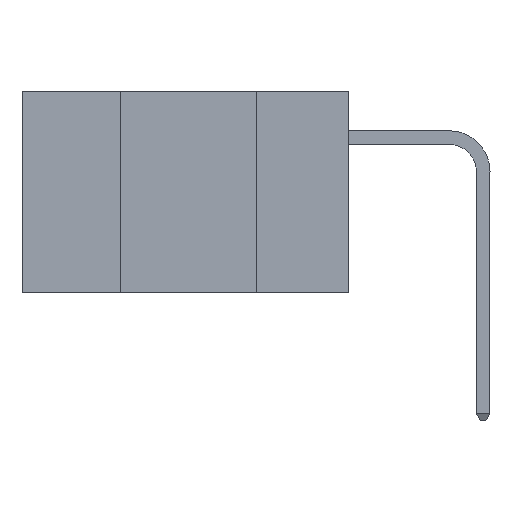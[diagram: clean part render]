
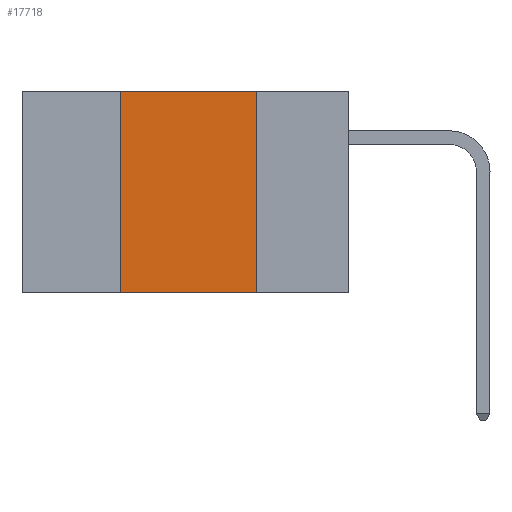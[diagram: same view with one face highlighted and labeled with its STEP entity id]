
A CAD part, left-side view. The second image highlights one B-rep face of the part: STEP entity #17718.
In plain terms, the highlighted planar face has unit normal (-1, 0, 0).
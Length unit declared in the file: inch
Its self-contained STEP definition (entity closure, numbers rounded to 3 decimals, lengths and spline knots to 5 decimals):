
#546 = VECTOR ( 'NONE', #20053, 39.37008 ) ;
#1324 = CARTESIAN_POINT ( 'NONE',  ( 0., 0.42, -0.37 ) ) ;
#2213 = DIRECTION ( 'NONE',  ( 0., 0., -1. ) ) ;
#2641 = DIRECTION ( 'NONE',  ( 1., 0., 0. ) ) ;
#4408 = EDGE_CURVE ( 'NONE', #5463, #21614, #23277, .T. ) ;
#4791 = AXIS2_PLACEMENT_3D ( 'NONE', #30560, #2641, #22536 ) ;
#4870 = EDGE_CURVE ( 'NONE', #34870, #12970, #35167, .T. ) ;
#5463 = VERTEX_POINT ( 'NONE', #24664 ) ;
#8190 = ORIENTED_EDGE ( 'NONE', *, *, #4870, .T. ) ;
#8892 = CARTESIAN_POINT ( 'NONE',  ( 0., 0.6, 0. ) ) ;
#10855 = DIRECTION ( 'NONE',  ( 0., -1., 0. ) ) ;
#12970 = VERTEX_POINT ( 'NONE', #28705 ) ;
#13222 = VECTOR ( 'NONE', #10855, 39.37008 ) ;
#15279 = ORIENTED_EDGE ( 'NONE', *, *, #23764, .F. ) ;
#16393 = EDGE_CURVE ( 'NONE', #34870, #5463, #30608, .T. ) ;
#17718 = ADVANCED_FACE ( 'NONE', ( #19771 ), #36065, .F. ) ;
#19184 = CARTESIAN_POINT ( 'NONE',  ( 0., 0.6, -0.37 ) ) ;
#19771 = FACE_OUTER_BOUND ( 'NONE', #27599, .T. ) ;
#20053 = DIRECTION ( 'NONE',  ( 0., -1., 0. ) ) ;
#21614 = VERTEX_POINT ( 'NONE', #23567 ) ;
#22442 = LINE ( 'NONE', #27680, #29725 ) ;
#22536 = DIRECTION ( 'NONE',  ( 0., 0., -1. ) ) ;
#23277 = LINE ( 'NONE', #8892, #546 ) ;
#23567 = CARTESIAN_POINT ( 'NONE',  ( 0., 0.17, 0. ) ) ;
#23764 = EDGE_CURVE ( 'NONE', #21614, #12970, #22442, .T. ) ;
#24664 = CARTESIAN_POINT ( 'NONE',  ( 0., 0.42, 0. ) ) ;
#27599 = EDGE_LOOP ( 'NONE', ( #15279, #35027, #28261, #8190 ) ) ;
#27680 = CARTESIAN_POINT ( 'NONE',  ( 0., 0.17, 0. ) ) ;
#28042 = VECTOR ( 'NONE', #32875, 39.37008 ) ;
#28261 = ORIENTED_EDGE ( 'NONE', *, *, #16393, .F. ) ;
#28705 = CARTESIAN_POINT ( 'NONE',  ( 0., 0.17, -0.37 ) ) ;
#29725 = VECTOR ( 'NONE', #2213, 39.37008 ) ;
#30560 = CARTESIAN_POINT ( 'NONE',  ( 0., 0.6, 0. ) ) ;
#30608 = LINE ( 'NONE', #35452, #28042 ) ;
#32875 = DIRECTION ( 'NONE',  ( 0., 0., 1. ) ) ;
#34870 = VERTEX_POINT ( 'NONE', #1324 ) ;
#35027 = ORIENTED_EDGE ( 'NONE', *, *, #4408, .F. ) ;
#35167 = LINE ( 'NONE', #19184, #13222 ) ;
#35452 = CARTESIAN_POINT ( 'NONE',  ( 0., 0.42, 0. ) ) ;
#36065 = PLANE ( 'NONE',  #4791 ) ;
